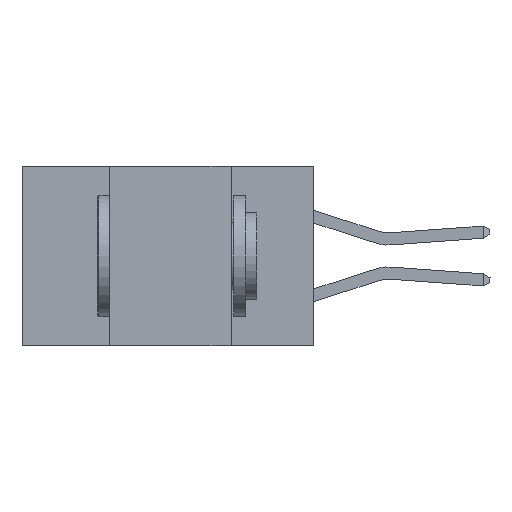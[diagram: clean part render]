
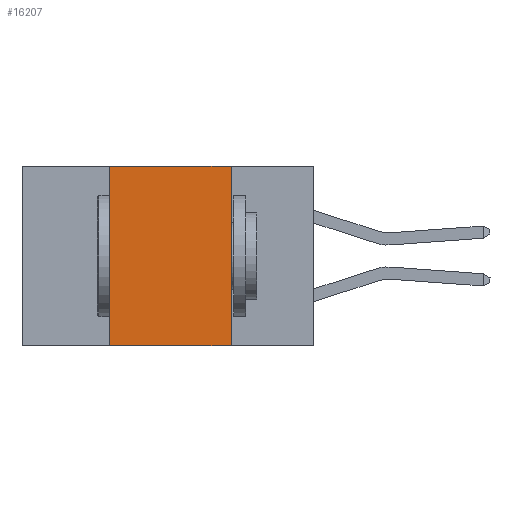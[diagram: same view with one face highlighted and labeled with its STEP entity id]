
A CAD part, left-side view. The second image highlights one B-rep face of the part: STEP entity #16207.
In plain terms, the highlighted planar face has unit normal (-1, 0, 0).
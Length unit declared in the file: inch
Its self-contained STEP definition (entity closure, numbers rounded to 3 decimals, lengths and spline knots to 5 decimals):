
#5 = EDGE_CURVE ( 'NONE', #4301, #15589, #551, .T. ) ;
#213 = CARTESIAN_POINT ( 'NONE',  ( 0., 0.42, -0.37 ) ) ;
#551 = LINE ( 'NONE', #15702, #5382 ) ;
#1962 = LINE ( 'NONE', #8435, #3258 ) ;
#2110 = VECTOR ( 'NONE', #11816, 39.37008 ) ;
#2250 = EDGE_CURVE ( 'NONE', #16577, #4578, #22371, .T. ) ;
#2428 = LINE ( 'NONE', #7925, #2110 ) ;
#2496 = DIRECTION ( 'NONE',  ( 0., -1., 0. ) ) ;
#3258 = VECTOR ( 'NONE', #2496, 39.37008 ) ;
#3299 = CARTESIAN_POINT ( 'NONE',  ( 0., 0.6, 0. ) ) ;
#4301 = VERTEX_POINT ( 'NONE', #25790 ) ;
#4578 = VERTEX_POINT ( 'NONE', #8082 ) ;
#4597 = VECTOR ( 'NONE', #13753, 39.37008 ) ;
#5358 = DIRECTION ( 'NONE',  ( 1., 0., 0. ) ) ;
#5382 = VECTOR ( 'NONE', #5686, 39.37008 ) ;
#5686 = DIRECTION ( 'NONE',  ( 0., 0., -1. ) ) ;
#5877 = CARTESIAN_POINT ( 'NONE',  ( 0., 0.42, 0. ) ) ;
#6215 = EDGE_CURVE ( 'NONE', #4578, #4301, #2428, .T. ) ;
#7925 = CARTESIAN_POINT ( 'NONE',  ( 0., 0.6, 0. ) ) ;
#8082 = CARTESIAN_POINT ( 'NONE',  ( 0., 0.42, 0. ) ) ;
#8435 = CARTESIAN_POINT ( 'NONE',  ( 0., 0.6, -0.37 ) ) ;
#10878 = EDGE_LOOP ( 'NONE', ( #16921, #20293, #20346, #20262 ) ) ;
#11264 = CARTESIAN_POINT ( 'NONE',  ( 0., 0.17, -0.37 ) ) ;
#11816 = DIRECTION ( 'NONE',  ( 0., -1., 0. ) ) ;
#13753 = DIRECTION ( 'NONE',  ( 0., 0., 1. ) ) ;
#15589 = VERTEX_POINT ( 'NONE', #11264 ) ;
#15702 = CARTESIAN_POINT ( 'NONE',  ( 0., 0.17, 0. ) ) ;
#15967 = EDGE_CURVE ( 'NONE', #16577, #15589, #1962, .T. ) ;
#16207 = ADVANCED_FACE ( 'NONE', ( #16765 ), #19541, .F. ) ;
#16577 = VERTEX_POINT ( 'NONE', #213 ) ;
#16765 = FACE_OUTER_BOUND ( 'NONE', #10878, .T. ) ;
#16921 = ORIENTED_EDGE ( 'NONE', *, *, #5, .F. ) ;
#19541 = PLANE ( 'NONE',  #22706 ) ;
#20262 = ORIENTED_EDGE ( 'NONE', *, *, #15967, .T. ) ;
#20293 = ORIENTED_EDGE ( 'NONE', *, *, #6215, .F. ) ;
#20346 = ORIENTED_EDGE ( 'NONE', *, *, #2250, .F. ) ;
#21514 = DIRECTION ( 'NONE',  ( 0., 0., -1. ) ) ;
#22371 = LINE ( 'NONE', #5877, #4597 ) ;
#22706 = AXIS2_PLACEMENT_3D ( 'NONE', #3299, #5358, #21514 ) ;
#25790 = CARTESIAN_POINT ( 'NONE',  ( 0., 0.17, 0. ) ) ;
